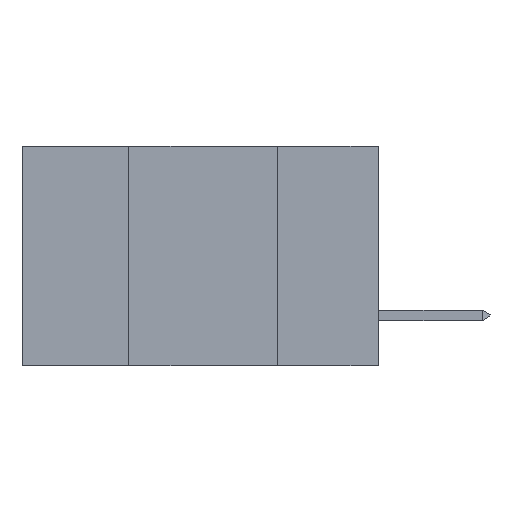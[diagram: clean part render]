
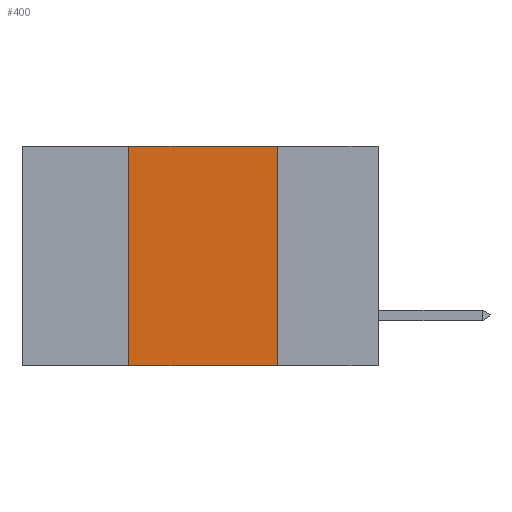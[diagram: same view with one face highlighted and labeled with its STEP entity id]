
A CAD part, left-side view. The second image highlights one B-rep face of the part: STEP entity #400.
In plain terms, the highlighted planar face has unit normal (-1, 0, 0).
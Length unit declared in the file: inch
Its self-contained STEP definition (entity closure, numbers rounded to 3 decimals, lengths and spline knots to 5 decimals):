
#400 = ADVANCED_FACE ( 'NONE', ( #15257 ), #2983, .F. ) ;
#553 = DIRECTION ( 'NONE',  ( 0., 0., -1. ) ) ;
#1709 = DIRECTION ( 'NONE',  ( 0., 0., 1. ) ) ;
#2257 = CARTESIAN_POINT ( 'NONE',  ( 0., 0.17, -0.37 ) ) ;
#2353 = ORIENTED_EDGE ( 'NONE', *, *, #13870, .F. ) ;
#2845 = EDGE_CURVE ( 'NONE', #9732, #14987, #16363, .T. ) ;
#2983 = PLANE ( 'NONE',  #9332 ) ;
#3044 = EDGE_CURVE ( 'NONE', #14987, #15230, #8970, .T. ) ;
#3674 = CARTESIAN_POINT ( 'NONE',  ( 0., 0.6, 0. ) ) ;
#4333 = VECTOR ( 'NONE', #9164, 39.37008 ) ;
#4557 = EDGE_LOOP ( 'NONE', ( #16908, #17303, #2353, #12967 ) ) ;
#5557 = EDGE_CURVE ( 'NONE', #12797, #15230, #6388, .T. ) ;
#5636 = CARTESIAN_POINT ( 'NONE',  ( 0., 0.42, -0.37 ) ) ;
#6388 = LINE ( 'NONE', #11841, #4333 ) ;
#6978 = LINE ( 'NONE', #5636, #16733 ) ;
#8970 = LINE ( 'NONE', #2257, #15762 ) ;
#9164 = DIRECTION ( 'NONE',  ( 0., -1., 0. ) ) ;
#9253 = CARTESIAN_POINT ( 'NONE',  ( 0., 0.6, 0. ) ) ;
#9332 = AXIS2_PLACEMENT_3D ( 'NONE', #3674, #14627, #553 ) ;
#9732 = VERTEX_POINT ( 'NONE', #12171 ) ;
#10210 = CARTESIAN_POINT ( 'NONE',  ( 0., 0.42, -0.37 ) ) ;
#11841 = CARTESIAN_POINT ( 'NONE',  ( 0., 0.6, -0.37 ) ) ;
#12171 = CARTESIAN_POINT ( 'NONE',  ( 0., 0.42, 0. ) ) ;
#12187 = CARTESIAN_POINT ( 'NONE',  ( 0., 0.17, 0. ) ) ;
#12797 = VERTEX_POINT ( 'NONE', #10210 ) ;
#12870 = VECTOR ( 'NONE', #17724, 39.37008 ) ;
#12967 = ORIENTED_EDGE ( 'NONE', *, *, #5557, .T. ) ;
#12997 = DIRECTION ( 'NONE',  ( 0., 0., -1. ) ) ;
#13068 = CARTESIAN_POINT ( 'NONE',  ( 0., 0.17, -0.37 ) ) ;
#13870 = EDGE_CURVE ( 'NONE', #12797, #9732, #6978, .T. ) ;
#14627 = DIRECTION ( 'NONE',  ( 1., 0., 0. ) ) ;
#14987 = VERTEX_POINT ( 'NONE', #12187 ) ;
#15230 = VERTEX_POINT ( 'NONE', #13068 ) ;
#15257 = FACE_OUTER_BOUND ( 'NONE', #4557, .T. ) ;
#15762 = VECTOR ( 'NONE', #12997, 39.37008 ) ;
#16363 = LINE ( 'NONE', #9253, #12870 ) ;
#16733 = VECTOR ( 'NONE', #1709, 39.37008 ) ;
#16908 = ORIENTED_EDGE ( 'NONE', *, *, #3044, .F. ) ;
#17303 = ORIENTED_EDGE ( 'NONE', *, *, #2845, .F. ) ;
#17724 = DIRECTION ( 'NONE',  ( 0., -1., 0. ) ) ;
